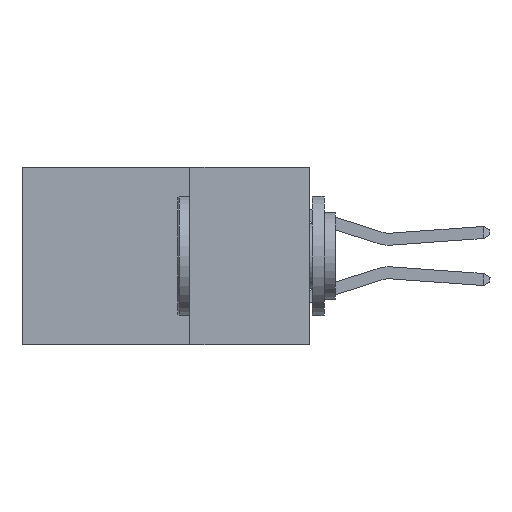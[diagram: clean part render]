
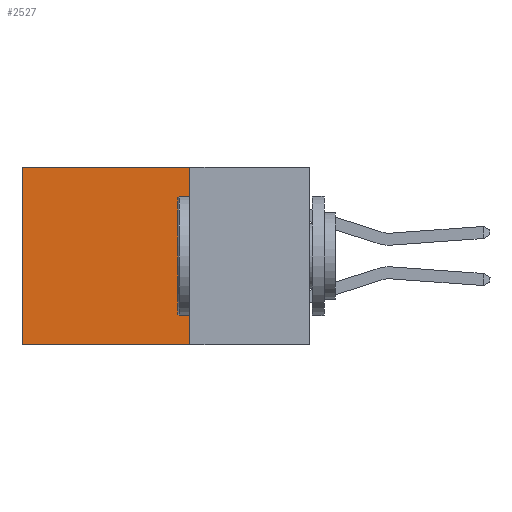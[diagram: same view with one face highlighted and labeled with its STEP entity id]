
A CAD part, left-side view. The second image highlights one B-rep face of the part: STEP entity #2527.
In plain terms, the highlighted planar face has unit normal (-1, 0, 0).
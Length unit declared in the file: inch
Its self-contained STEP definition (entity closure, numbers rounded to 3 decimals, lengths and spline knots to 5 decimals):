
#874 = LINE ( 'NONE', #2644, #4561 ) ;
#2473 = CARTESIAN_POINT ( 'NONE',  ( 0.2615, 0.6, 0. ) ) ;
#2527 = ADVANCED_FACE ( 'NONE', ( #4817 ), #10685, .F. ) ;
#2644 = CARTESIAN_POINT ( 'NONE',  ( 0.2615, 0.25, -0.37 ) ) ;
#2841 = DIRECTION ( 'NONE',  ( 0., 0., -1. ) ) ;
#3599 = VECTOR ( 'NONE', #4311, 39.37008 ) ;
#3978 = VERTEX_POINT ( 'NONE', #4071 ) ;
#4013 = LINE ( 'NONE', #12354, #3599 ) ;
#4071 = CARTESIAN_POINT ( 'NONE',  ( 0.2615, 0.25, 0. ) ) ;
#4311 = DIRECTION ( 'NONE',  ( 0., 0., -1. ) ) ;
#4560 = ORIENTED_EDGE ( 'NONE', *, *, #10590, .F. ) ;
#4561 = VECTOR ( 'NONE', #2841, 39.37008 ) ;
#4817 = FACE_OUTER_BOUND ( 'NONE', #9866, .T. ) ;
#5188 = EDGE_CURVE ( 'NONE', #3978, #12606, #874, .T. ) ;
#6660 = CARTESIAN_POINT ( 'NONE',  ( 0.2615, 0.6, -0.37 ) ) ;
#7379 = DIRECTION ( 'NONE',  ( 0., 1., 0. ) ) ;
#8439 = VECTOR ( 'NONE', #14609, 39.37008 ) ;
#8480 = EDGE_CURVE ( 'NONE', #3978, #11321, #15582, .T. ) ;
#9023 = LINE ( 'NONE', #11405, #16118 ) ;
#9659 = ORIENTED_EDGE ( 'NONE', *, *, #10010, .T. ) ;
#9866 = EDGE_LOOP ( 'NONE', ( #9659, #4560, #12236, #12211 ) ) ;
#10010 = EDGE_CURVE ( 'NONE', #11321, #13411, #4013, .T. ) ;
#10590 = EDGE_CURVE ( 'NONE', #12606, #13411, #9023, .T. ) ;
#10630 = DIRECTION ( 'NONE',  ( 1., 0., 0. ) ) ;
#10646 = DIRECTION ( 'NONE',  ( 0., 0., -1. ) ) ;
#10685 = PLANE ( 'NONE',  #16022 ) ;
#10717 = CARTESIAN_POINT ( 'NONE',  ( 0.2615, 0.25, -0.37 ) ) ;
#11321 = VERTEX_POINT ( 'NONE', #2473 ) ;
#11405 = CARTESIAN_POINT ( 'NONE',  ( 0.2615, 0.25, -0.37 ) ) ;
#12211 = ORIENTED_EDGE ( 'NONE', *, *, #8480, .T. ) ;
#12236 = ORIENTED_EDGE ( 'NONE', *, *, #5188, .F. ) ;
#12354 = CARTESIAN_POINT ( 'NONE',  ( 0.2615, 0.6, -0.37 ) ) ;
#12606 = VERTEX_POINT ( 'NONE', #13088 ) ;
#13088 = CARTESIAN_POINT ( 'NONE',  ( 0.2615, 0.25, -0.37 ) ) ;
#13272 = CARTESIAN_POINT ( 'NONE',  ( 0.2615, 0.25, 0. ) ) ;
#13411 = VERTEX_POINT ( 'NONE', #6660 ) ;
#14609 = DIRECTION ( 'NONE',  ( 0., 1., 0. ) ) ;
#15582 = LINE ( 'NONE', #13272, #8439 ) ;
#16022 = AXIS2_PLACEMENT_3D ( 'NONE', #10717, #10630, #10646 ) ;
#16118 = VECTOR ( 'NONE', #7379, 39.37008 ) ;
